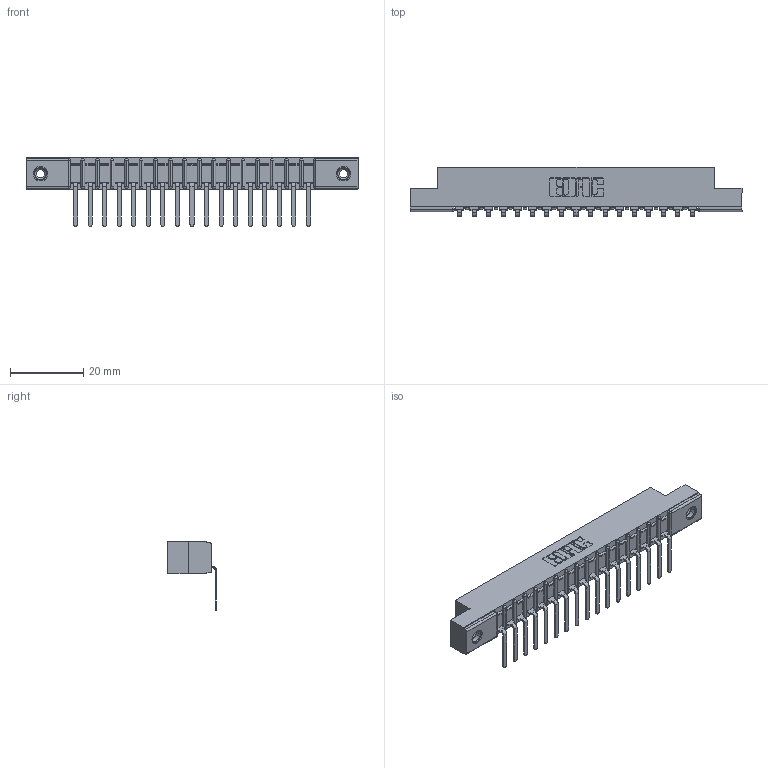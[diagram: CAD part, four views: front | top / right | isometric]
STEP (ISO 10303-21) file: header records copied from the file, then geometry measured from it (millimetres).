
FILE_DESCRIPTION (( 'STEP AP203' ), '1' );
FILE_NAME ('307-017-457-108.STEP', '2020-09-25T22:40:59', ( '' ), ( '' ), 'SwSTEP 2.0', 'SolidWorks 2020', '' );
FILE_SCHEMA (( 'CONFIG_CONTROL_DESIGN' ));
Length unit declared in the file: inch
Products named in the file (4): 307 Part_.156 Dia Mounting Holes; 307-017-457-108; 345-250-001_345-250-003-102; 307-290-002_557
Assembly tree (20 placements, depth 2):
  307-017-457-108
    307 Part_.156 Dia Mounting Holes
    307-290-002_557  x17
    345-250-001_345-250-003-102  x2
Bounding box: 90.37 x 13.32 x 18.67 mm (x, y, z)
Volume: 6003 mm3; surface area: 10939.5 mm2
Topology: 20 solids, 20 shells, 1522 faces, 4607 edges, 3014 vertices
Faces by surface type: plane 901, cylinder 569, sphere 36, cone 12, torus 4
Entity records: 19695 total; most frequent: CARTESIAN_POINT 3299, ORIENTED_EDGE 3282, DIRECTION 3227, EDGE_CURVE 1641, VECTOR 1243, LINE 1243, VERTEX_POINT 1064, AXIS2_PLACEMENT_3D 992
